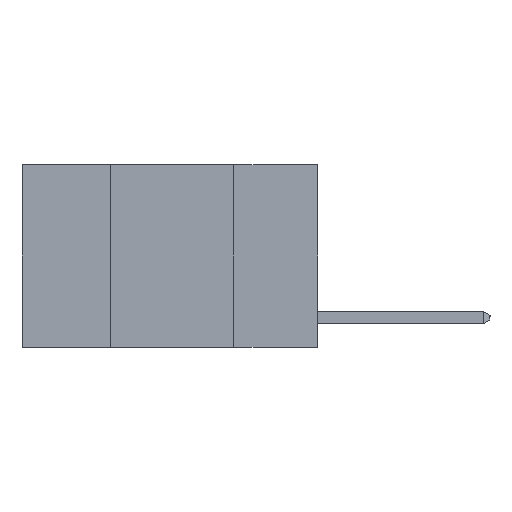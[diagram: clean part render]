
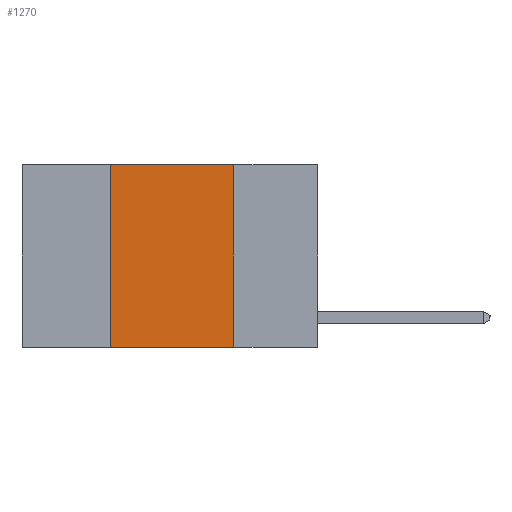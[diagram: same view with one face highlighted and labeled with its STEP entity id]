
A CAD part, left-side view. The second image highlights one B-rep face of the part: STEP entity #1270.
In plain terms, the highlighted planar face has unit normal (-1, 0, 0).
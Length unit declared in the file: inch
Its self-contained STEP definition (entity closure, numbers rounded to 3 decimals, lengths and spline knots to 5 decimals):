
#205 = VECTOR ( 'NONE', #14971, 39.37008 ) ;
#951 = VERTEX_POINT ( 'NONE', #5984 ) ;
#1270 = ADVANCED_FACE ( 'NONE', ( #11982 ), #9730, .F. ) ;
#2166 = ORIENTED_EDGE ( 'NONE', *, *, #6314, .F. ) ;
#3566 = ORIENTED_EDGE ( 'NONE', *, *, #5540, .F. ) ;
#3631 = CARTESIAN_POINT ( 'NONE',  ( 0., 0.6, -0.37 ) ) ;
#3762 = LINE ( 'NONE', #6630, #9927 ) ;
#4726 = EDGE_CURVE ( 'NONE', #5331, #5680, #5744, .T. ) ;
#4848 = CARTESIAN_POINT ( 'NONE',  ( 0., 0.6, 0. ) ) ;
#5331 = VERTEX_POINT ( 'NONE', #6058 ) ;
#5540 = EDGE_CURVE ( 'NONE', #5331, #951, #7254, .T. ) ;
#5680 = VERTEX_POINT ( 'NONE', #15251 ) ;
#5744 = LINE ( 'NONE', #3631, #15121 ) ;
#5984 = CARTESIAN_POINT ( 'NONE',  ( 0., 0.42, 0. ) ) ;
#6058 = CARTESIAN_POINT ( 'NONE',  ( 0., 0.42, -0.37 ) ) ;
#6076 = DIRECTION ( 'NONE',  ( 1., 0., 0. ) ) ;
#6314 = EDGE_CURVE ( 'NONE', #951, #15098, #13558, .T. ) ;
#6365 = EDGE_CURVE ( 'NONE', #15098, #5680, #3762, .T. ) ;
#6630 = CARTESIAN_POINT ( 'NONE',  ( 0., 0.17, 0. ) ) ;
#7254 = LINE ( 'NONE', #13771, #205 ) ;
#7425 = VECTOR ( 'NONE', #13854, 39.37008 ) ;
#7872 = DIRECTION ( 'NONE',  ( 0., 0., -1. ) ) ;
#8765 = ORIENTED_EDGE ( 'NONE', *, *, #4726, .T. ) ;
#9730 = PLANE ( 'NONE',  #15501 ) ;
#9927 = VECTOR ( 'NONE', #7872, 39.37008 ) ;
#10523 = EDGE_LOOP ( 'NONE', ( #11642, #2166, #3566, #8765 ) ) ;
#11453 = CARTESIAN_POINT ( 'NONE',  ( 0., 0.6, 0. ) ) ;
#11642 = ORIENTED_EDGE ( 'NONE', *, *, #6365, .F. ) ;
#11982 = FACE_OUTER_BOUND ( 'NONE', #10523, .T. ) ;
#13558 = LINE ( 'NONE', #11453, #7425 ) ;
#13771 = CARTESIAN_POINT ( 'NONE',  ( 0., 0.42, 0. ) ) ;
#13854 = DIRECTION ( 'NONE',  ( 0., -1., 0. ) ) ;
#14301 = CARTESIAN_POINT ( 'NONE',  ( 0., 0.17, 0. ) ) ;
#14612 = DIRECTION ( 'NONE',  ( 0., 0., -1. ) ) ;
#14971 = DIRECTION ( 'NONE',  ( 0., 0., 1. ) ) ;
#15098 = VERTEX_POINT ( 'NONE', #14301 ) ;
#15121 = VECTOR ( 'NONE', #15893, 39.37008 ) ;
#15251 = CARTESIAN_POINT ( 'NONE',  ( 0., 0.17, -0.37 ) ) ;
#15501 = AXIS2_PLACEMENT_3D ( 'NONE', #4848, #6076, #14612 ) ;
#15893 = DIRECTION ( 'NONE',  ( 0., -1., 0. ) ) ;
